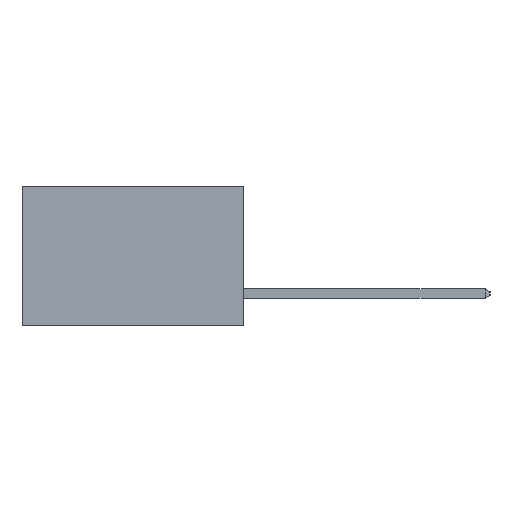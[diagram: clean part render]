
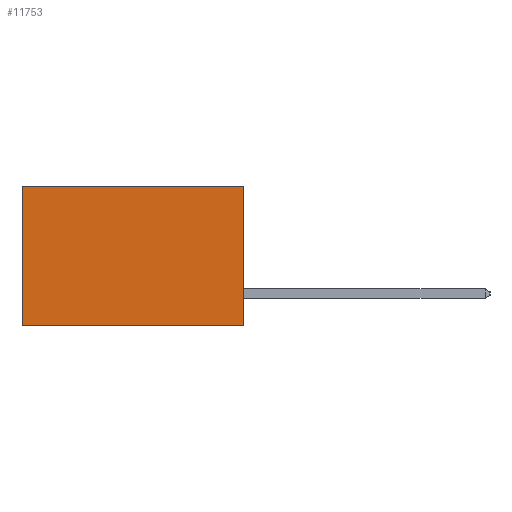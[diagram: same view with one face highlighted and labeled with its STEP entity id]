
A CAD part, left-side view. The second image highlights one B-rep face of the part: STEP entity #11753.
In plain terms, the highlighted planar face has unit normal (-1, 0, 0).
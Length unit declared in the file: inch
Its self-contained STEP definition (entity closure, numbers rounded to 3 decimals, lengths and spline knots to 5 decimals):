
#526 = AXIS2_PLACEMENT_3D ( 'NONE', #9953, #3378, #11016 ) ;
#586 = VERTEX_POINT ( 'NONE', #6987 ) ;
#1012 = FACE_OUTER_BOUND ( 'NONE', #9986, .T. ) ;
#1136 = LINE ( 'NONE', #8980, #2268 ) ;
#1784 = DIRECTION ( 'NONE',  ( 0., 0., -1. ) ) ;
#2187 = VERTEX_POINT ( 'NONE', #2896 ) ;
#2268 = VECTOR ( 'NONE', #12165, 39.37008 ) ;
#2772 = VECTOR ( 'NONE', #11953, 39.37008 ) ;
#2896 = CARTESIAN_POINT ( 'NONE',  ( 0.277, 0.59, 0. ) ) ;
#3250 = EDGE_CURVE ( 'NONE', #9617, #586, #11513, .T. ) ;
#3336 = EDGE_CURVE ( 'NONE', #13650, #2187, #10511, .T. ) ;
#3378 = DIRECTION ( 'NONE',  ( 1., 0., 0. ) ) ;
#4024 = VECTOR ( 'NONE', #6185, 39.37008 ) ;
#5214 = CARTESIAN_POINT ( 'NONE',  ( 0.277, 0.59, -0.37 ) ) ;
#6185 = DIRECTION ( 'NONE',  ( 0., 1., 0. ) ) ;
#6728 = LINE ( 'NONE', #5214, #12410 ) ;
#6987 = CARTESIAN_POINT ( 'NONE',  ( 0.277, 0.59, -0.37 ) ) ;
#7778 = PLANE ( 'NONE',  #526 ) ;
#8980 = CARTESIAN_POINT ( 'NONE',  ( 0.277, 0., -0.37 ) ) ;
#9336 = ORIENTED_EDGE ( 'NONE', *, *, #3250, .F. ) ;
#9617 = VERTEX_POINT ( 'NONE', #9952 ) ;
#9679 = ORIENTED_EDGE ( 'NONE', *, *, #13611, .F. ) ;
#9952 = CARTESIAN_POINT ( 'NONE',  ( 0.277, 0., -0.37 ) ) ;
#9953 = CARTESIAN_POINT ( 'NONE',  ( 0.277, 0., -0.37 ) ) ;
#9986 = EDGE_LOOP ( 'NONE', ( #12442, #9336, #9679, #10657 ) ) ;
#10511 = LINE ( 'NONE', #10632, #4024 ) ;
#10632 = CARTESIAN_POINT ( 'NONE',  ( 0.277, 0., 0. ) ) ;
#10657 = ORIENTED_EDGE ( 'NONE', *, *, #3336, .T. ) ;
#11016 = DIRECTION ( 'NONE',  ( 0., 0., -1. ) ) ;
#11155 = CARTESIAN_POINT ( 'NONE',  ( 0.277, 0., 0. ) ) ;
#11513 = LINE ( 'NONE', #11992, #2772 ) ;
#11753 = ADVANCED_FACE ( 'NONE', ( #1012 ), #7778, .F. ) ;
#11953 = DIRECTION ( 'NONE',  ( 0., 1., 0. ) ) ;
#11992 = CARTESIAN_POINT ( 'NONE',  ( 0.277, 0., -0.37 ) ) ;
#12164 = EDGE_CURVE ( 'NONE', #2187, #586, #6728, .T. ) ;
#12165 = DIRECTION ( 'NONE',  ( 0., 0., -1. ) ) ;
#12410 = VECTOR ( 'NONE', #1784, 39.37008 ) ;
#12442 = ORIENTED_EDGE ( 'NONE', *, *, #12164, .T. ) ;
#13611 = EDGE_CURVE ( 'NONE', #13650, #9617, #1136, .T. ) ;
#13650 = VERTEX_POINT ( 'NONE', #11155 ) ;
